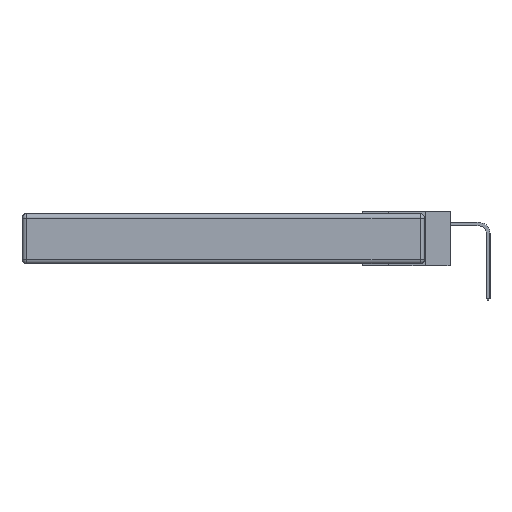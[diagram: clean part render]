
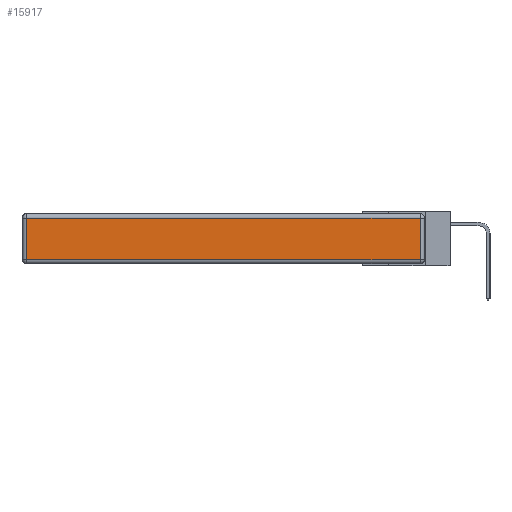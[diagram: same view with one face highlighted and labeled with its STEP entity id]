
A CAD part, left-side view. The second image highlights one B-rep face of the part: STEP entity #15917.
In plain terms, the highlighted planar face has unit normal (-1, 0, 0).
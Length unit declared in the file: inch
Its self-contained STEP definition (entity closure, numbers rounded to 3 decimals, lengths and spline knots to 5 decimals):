
#236 = DIRECTION ( 'NONE',  ( 0., 0., -1. ) ) ;
#1765 = DIRECTION ( 'NONE',  ( 0., 1., 0. ) ) ;
#3114 = VERTEX_POINT ( 'NONE', #34338 ) ;
#3506 = EDGE_CURVE ( 'NONE', #9973, #16949, #30807, .T. ) ;
#5678 = CARTESIAN_POINT ( 'NONE',  ( 0., 0.03, -0.343 ) ) ;
#5797 = VECTOR ( 'NONE', #33946, 39.37008 ) ;
#7339 = PLANE ( 'NONE',  #17262 ) ;
#8467 = CARTESIAN_POINT ( 'NONE',  ( 0., 2.72, -0.343 ) ) ;
#8659 = VECTOR ( 'NONE', #29879, 39.37008 ) ;
#9516 = LINE ( 'NONE', #5678, #8659 ) ;
#9973 = VERTEX_POINT ( 'NONE', #25089 ) ;
#10056 = CARTESIAN_POINT ( 'NONE',  ( 0., 0., -0.343 ) ) ;
#11843 = ORIENTED_EDGE ( 'NONE', *, *, #17934, .T. ) ;
#12780 = DIRECTION ( 'NONE',  ( 0., 0., 1. ) ) ;
#12945 = LINE ( 'NONE', #25883, #5797 ) ;
#14270 = ORIENTED_EDGE ( 'NONE', *, *, #21566, .T. ) ;
#15917 = ADVANCED_FACE ( 'NONE', ( #18393 ), #7339, .T. ) ;
#16949 = VERTEX_POINT ( 'NONE', #22832 ) ;
#17262 = AXIS2_PLACEMENT_3D ( 'NONE', #10056, #18900, #12780 ) ;
#17791 = VECTOR ( 'NONE', #1765, 39.37008 ) ;
#17934 = EDGE_CURVE ( 'NONE', #16949, #3114, #22444, .T. ) ;
#18393 = FACE_OUTER_BOUND ( 'NONE', #24626, .T. ) ;
#18632 = ORIENTED_EDGE ( 'NONE', *, *, #24291, .T. ) ;
#18900 = DIRECTION ( 'NONE',  ( -1., 0., 0. ) ) ;
#19925 = CARTESIAN_POINT ( 'NONE',  ( 0., 2.75, -0.03 ) ) ;
#21566 = EDGE_CURVE ( 'NONE', #3114, #32623, #12945, .T. ) ;
#22444 = LINE ( 'NONE', #8467, #32510 ) ;
#22832 = CARTESIAN_POINT ( 'NONE',  ( 0., 2.72, -0.03 ) ) ;
#24291 = EDGE_CURVE ( 'NONE', #32623, #9973, #9516, .T. ) ;
#24626 = EDGE_LOOP ( 'NONE', ( #14270, #18632, #28862, #11843 ) ) ;
#25089 = CARTESIAN_POINT ( 'NONE',  ( 0., 0.03, -0.03 ) ) ;
#25883 = CARTESIAN_POINT ( 'NONE',  ( 0., 0., -0.313 ) ) ;
#26091 = CARTESIAN_POINT ( 'NONE',  ( 0., 0.03, -0.313 ) ) ;
#28862 = ORIENTED_EDGE ( 'NONE', *, *, #3506, .T. ) ;
#29879 = DIRECTION ( 'NONE',  ( 0., 0., 1. ) ) ;
#30807 = LINE ( 'NONE', #19925, #17791 ) ;
#32510 = VECTOR ( 'NONE', #236, 39.37008 ) ;
#32623 = VERTEX_POINT ( 'NONE', #26091 ) ;
#33946 = DIRECTION ( 'NONE',  ( 0., -1., 0. ) ) ;
#34338 = CARTESIAN_POINT ( 'NONE',  ( 0., 2.72, -0.313 ) ) ;
